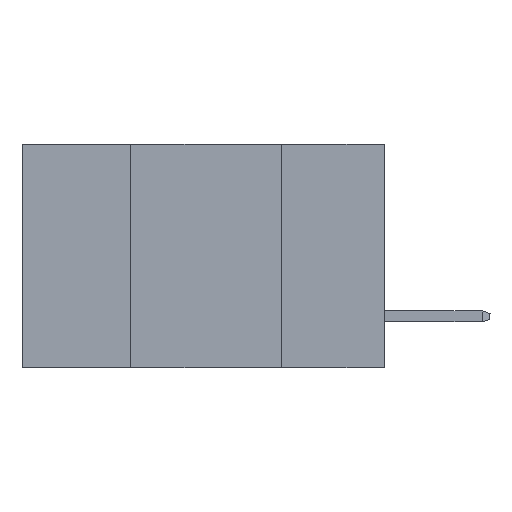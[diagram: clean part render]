
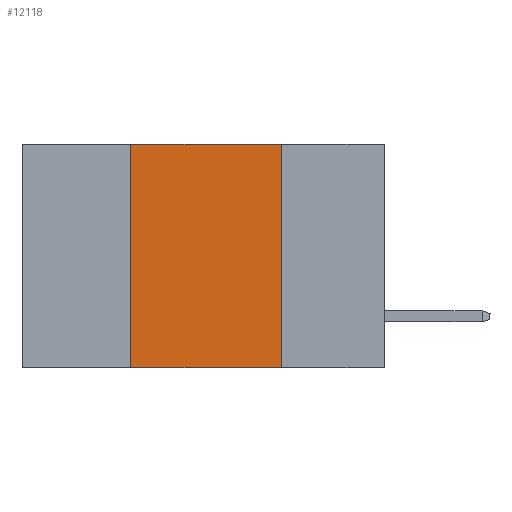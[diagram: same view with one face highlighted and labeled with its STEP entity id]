
A CAD part, left-side view. The second image highlights one B-rep face of the part: STEP entity #12118.
In plain terms, the highlighted planar face has unit normal (-1, 0, 0).
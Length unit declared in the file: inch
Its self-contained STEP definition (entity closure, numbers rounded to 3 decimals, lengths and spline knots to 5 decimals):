
#326 = DIRECTION ( 'NONE',  ( 0., 0., -1. ) ) ;
#390 = VECTOR ( 'NONE', #9130, 39.37008 ) ;
#810 = EDGE_CURVE ( 'NONE', #16689, #5587, #16772, .T. ) ;
#2142 = CARTESIAN_POINT ( 'NONE',  ( 0., 0.17, 0. ) ) ;
#4118 = CARTESIAN_POINT ( 'NONE',  ( 0., 0.17, 0. ) ) ;
#5587 = VERTEX_POINT ( 'NONE', #6430 ) ;
#5887 = DIRECTION ( 'NONE',  ( 0., -1., 0. ) ) ;
#5977 = VERTEX_POINT ( 'NONE', #11472 ) ;
#6430 = CARTESIAN_POINT ( 'NONE',  ( 0., 0.17, -0.37 ) ) ;
#6940 = DIRECTION ( 'NONE',  ( 0., -1., 0. ) ) ;
#7669 = EDGE_CURVE ( 'NONE', #12877, #5587, #9788, .T. ) ;
#7847 = EDGE_LOOP ( 'NONE', ( #10710, #13750, #9406, #12979 ) ) ;
#9130 = DIRECTION ( 'NONE',  ( 0., 0., 1. ) ) ;
#9406 = ORIENTED_EDGE ( 'NONE', *, *, #10699, .F. ) ;
#9538 = CARTESIAN_POINT ( 'NONE',  ( 0., 0.6, -0.37 ) ) ;
#9733 = EDGE_CURVE ( 'NONE', #5977, #16689, #16775, .T. ) ;
#9775 = PLANE ( 'NONE',  #15694 ) ;
#9788 = LINE ( 'NONE', #9538, #16035 ) ;
#10613 = FACE_OUTER_BOUND ( 'NONE', #7847, .T. ) ;
#10699 = EDGE_CURVE ( 'NONE', #12877, #5977, #15651, .T. ) ;
#10710 = ORIENTED_EDGE ( 'NONE', *, *, #810, .F. ) ;
#11472 = CARTESIAN_POINT ( 'NONE',  ( 0., 0.42, 0. ) ) ;
#11521 = DIRECTION ( 'NONE',  ( 0., 0., -1. ) ) ;
#12009 = VECTOR ( 'NONE', #5887, 39.37008 ) ;
#12118 = ADVANCED_FACE ( 'NONE', ( #10613 ), #9775, .F. ) ;
#12877 = VERTEX_POINT ( 'NONE', #17180 ) ;
#12979 = ORIENTED_EDGE ( 'NONE', *, *, #7669, .T. ) ;
#13750 = ORIENTED_EDGE ( 'NONE', *, *, #9733, .F. ) ;
#13780 = CARTESIAN_POINT ( 'NONE',  ( 0., 0.6, 0. ) ) ;
#13794 = CARTESIAN_POINT ( 'NONE',  ( 0., 0.6, 0. ) ) ;
#15132 = DIRECTION ( 'NONE',  ( 1., 0., 0. ) ) ;
#15543 = VECTOR ( 'NONE', #11521, 39.37008 ) ;
#15651 = LINE ( 'NONE', #16006, #390 ) ;
#15694 = AXIS2_PLACEMENT_3D ( 'NONE', #13794, #15132, #326 ) ;
#16006 = CARTESIAN_POINT ( 'NONE',  ( 0., 0.42, 0. ) ) ;
#16035 = VECTOR ( 'NONE', #6940, 39.37008 ) ;
#16689 = VERTEX_POINT ( 'NONE', #4118 ) ;
#16772 = LINE ( 'NONE', #2142, #15543 ) ;
#16775 = LINE ( 'NONE', #13780, #12009 ) ;
#17180 = CARTESIAN_POINT ( 'NONE',  ( 0., 0.42, -0.37 ) ) ;
